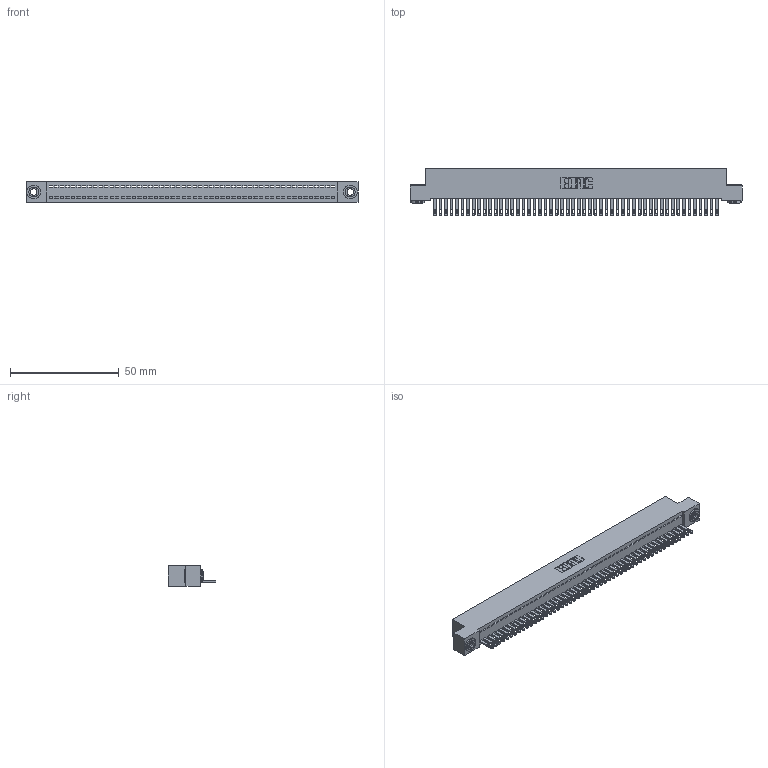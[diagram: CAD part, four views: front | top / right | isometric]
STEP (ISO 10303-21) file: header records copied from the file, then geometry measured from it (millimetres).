
FILE_DESCRIPTION (( 'STEP AP203' ), '1' );
FILE_NAME ('342-052-500-103.STEP', '2018-08-12T21:17:32', ( '' ), ( '' ), 'SwSTEP 2.0', 'SolidWorks 2016', '' );
FILE_SCHEMA (( 'CONFIG_CONTROL_DESIGN' ));
Length unit declared in the file: inch
Products named in the file (4): 342 Part_.156 TH; 345-292-001_345-293-100; 342-250-002_345-250-002-102; 342-052-500-103
Assembly tree (55 placements, depth 2):
  342-052-500-103
    342 Part_.156 TH
    345-292-001_345-293-100  x52
    342-250-002_345-250-002-102  x2
Bounding box: 152.4 x 21.85 x 9.4 mm (x, y, z)
Volume: 13454.3 mm3; surface area: 20272.2 mm2
Topology: 55 solids, 55 shells, 2956 faces, 9111 edges, 6070 vertices
Faces by surface type: plane 1948, cylinder 1000, cone 8
Entity records: 30944 total; most frequent: CARTESIAN_POINT 5313, ORIENTED_EDGE 5294, DIRECTION 4497, EDGE_CURVE 2647, VECTOR 2491, LINE 2491, VERTEX_POINT 1762, AXIS2_PLACEMENT_3D 1003
